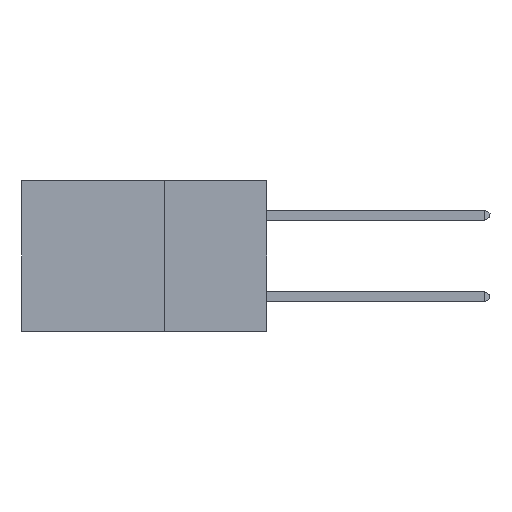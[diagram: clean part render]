
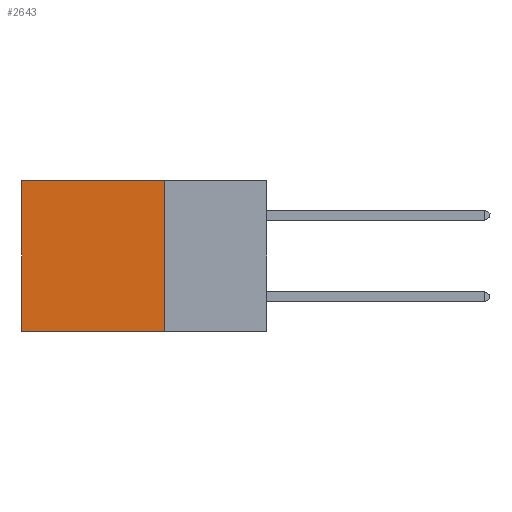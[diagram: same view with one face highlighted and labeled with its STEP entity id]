
A CAD part, left-side view. The second image highlights one B-rep face of the part: STEP entity #2643.
In plain terms, the highlighted planar face has unit normal (-1, 0, 0).
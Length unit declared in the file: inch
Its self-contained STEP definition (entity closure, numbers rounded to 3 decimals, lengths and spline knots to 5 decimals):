
#235 = LINE ( 'NONE', #1363, #9107 ) ;
#714 = EDGE_LOOP ( 'NONE', ( #4583, #16380, #3526, #13351 ) ) ;
#1006 = CARTESIAN_POINT ( 'NONE',  ( 0.2875, 0.6, 0. ) ) ;
#1363 = CARTESIAN_POINT ( 'NONE',  ( 0.2875, 0.25, 0. ) ) ;
#2486 = CARTESIAN_POINT ( 'NONE',  ( 0.2875, 0.25, -0.37 ) ) ;
#2643 = ADVANCED_FACE ( 'NONE', ( #6384 ), #11597, .F. ) ;
#2844 = CARTESIAN_POINT ( 'NONE',  ( 0.2875, 0.25, -0.37 ) ) ;
#2980 = VERTEX_POINT ( 'NONE', #8382 ) ;
#3284 = LINE ( 'NONE', #1006, #15210 ) ;
#3526 = ORIENTED_EDGE ( 'NONE', *, *, #13670, .F. ) ;
#4583 = ORIENTED_EDGE ( 'NONE', *, *, #16220, .T. ) ;
#6384 = FACE_OUTER_BOUND ( 'NONE', #714, .T. ) ;
#6978 = EDGE_CURVE ( 'NONE', #2980, #11582, #235, .T. ) ;
#7603 = DIRECTION ( 'NONE',  ( 0., 0., -1. ) ) ;
#7702 = VECTOR ( 'NONE', #10456, 39.37008 ) ;
#7730 = VECTOR ( 'NONE', #14384, 39.37008 ) ;
#8208 = CARTESIAN_POINT ( 'NONE',  ( 0.2875, 0.6, 0. ) ) ;
#8382 = CARTESIAN_POINT ( 'NONE',  ( 0.2875, 0.25, 0. ) ) ;
#9070 = CARTESIAN_POINT ( 'NONE',  ( 0.2875, 0.25, 0. ) ) ;
#9107 = VECTOR ( 'NONE', #9366, 39.37008 ) ;
#9366 = DIRECTION ( 'NONE',  ( 0., 1., 0. ) ) ;
#10456 = DIRECTION ( 'NONE',  ( 0., 0., -1. ) ) ;
#10486 = DIRECTION ( 'NONE',  ( 0., 0., -1. ) ) ;
#11513 = CARTESIAN_POINT ( 'NONE',  ( 0.2875, 0.25, 0. ) ) ;
#11582 = VERTEX_POINT ( 'NONE', #8208 ) ;
#11597 = PLANE ( 'NONE',  #13424 ) ;
#11680 = DIRECTION ( 'NONE',  ( 1., 0., 0. ) ) ;
#12853 = CARTESIAN_POINT ( 'NONE',  ( 0.2875, 0.6, -0.37 ) ) ;
#13351 = ORIENTED_EDGE ( 'NONE', *, *, #6978, .T. ) ;
#13424 = AXIS2_PLACEMENT_3D ( 'NONE', #11513, #11680, #7603 ) ;
#13670 = EDGE_CURVE ( 'NONE', #2980, #16425, #15746, .T. ) ;
#14384 = DIRECTION ( 'NONE',  ( 0., 1., 0. ) ) ;
#15210 = VECTOR ( 'NONE', #10486, 39.37008 ) ;
#15746 = LINE ( 'NONE', #9070, #7702 ) ;
#15750 = VERTEX_POINT ( 'NONE', #12853 ) ;
#15771 = LINE ( 'NONE', #2486, #7730 ) ;
#16220 = EDGE_CURVE ( 'NONE', #11582, #15750, #3284, .T. ) ;
#16221 = EDGE_CURVE ( 'NONE', #16425, #15750, #15771, .T. ) ;
#16380 = ORIENTED_EDGE ( 'NONE', *, *, #16221, .F. ) ;
#16425 = VERTEX_POINT ( 'NONE', #2844 ) ;
